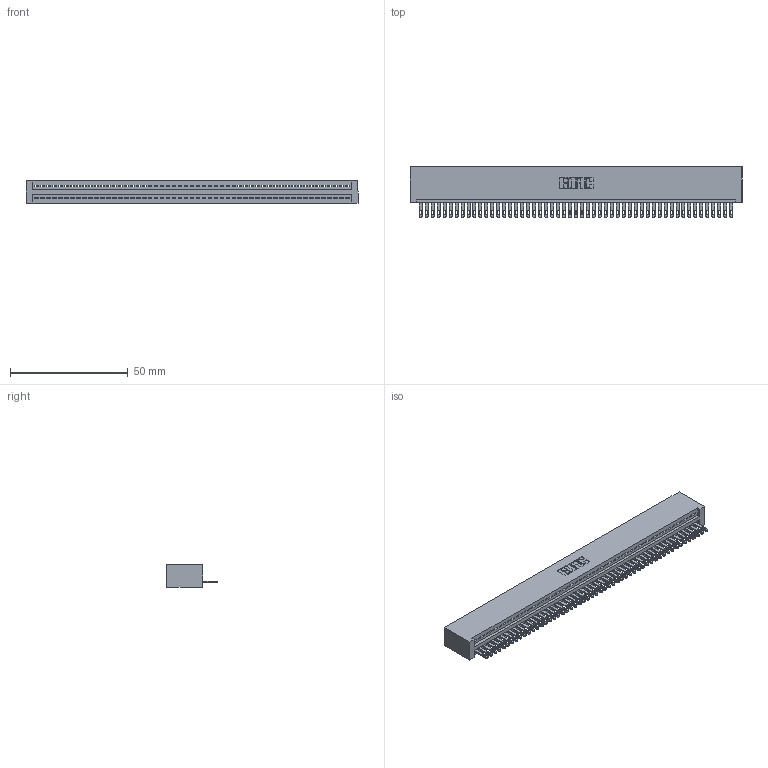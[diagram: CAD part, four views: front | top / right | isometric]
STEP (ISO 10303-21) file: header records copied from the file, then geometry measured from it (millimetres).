
FILE_DESCRIPTION (( 'STEP AP203' ), '1' );
FILE_NAME ('345-053-500-101.STEP', '2018-09-23T16:29:56', ( '' ), ( '' ), 'SwSTEP 2.0', 'SolidWorks 2016', '' );
FILE_SCHEMA (( 'CONFIG_CONTROL_DESIGN' ));
Length unit declared in the file: inch
Products named in the file (3): 345 Part_No Mounting Lugs; 345-292-001_345-293-100; 345-053-500-101
Assembly tree (54 placements, depth 2):
  345-053-500-101
    345 Part_No Mounting Lugs
    345-292-001_345-293-100  x53
Bounding box: 141.22 x 21.51 x 9.4 mm (x, y, z)
Volume: 14120.9 mm3; surface area: 19224 mm2
Topology: 54 solids, 54 shells, 2980 faces, 9221 edges, 6146 vertices
Faces by surface type: plane 1878, cylinder 1102
Entity records: 38061 total; most frequent: CARTESIAN_POINT 6599, ORIENTED_EDGE 6586, DIRECTION 5743, EDGE_CURVE 3293, VECTOR 2953, LINE 2953, VERTEX_POINT 2194, AXIS2_PLACEMENT_3D 1395
